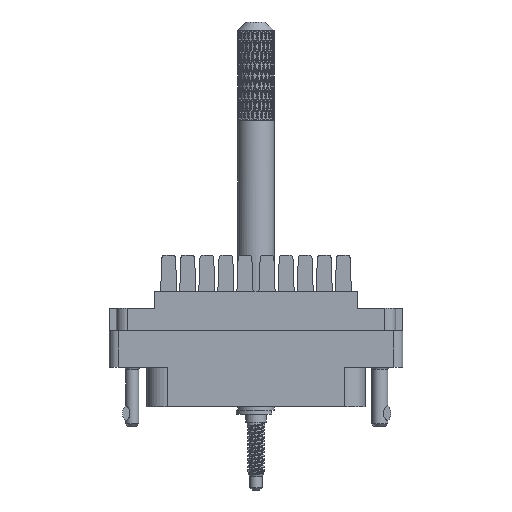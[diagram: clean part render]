
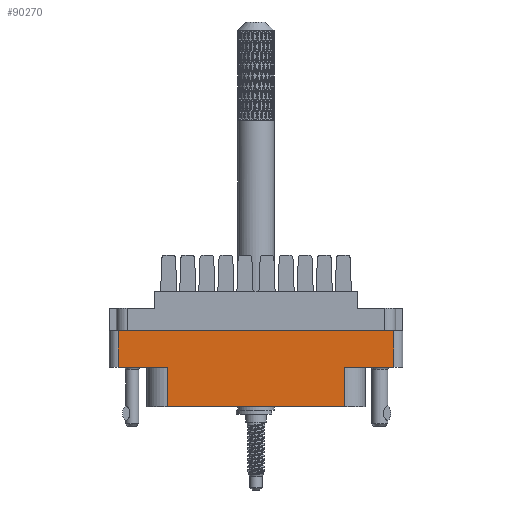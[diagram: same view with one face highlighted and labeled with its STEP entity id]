
A CAD part, front view. The second image highlights one B-rep face of the part: STEP entity #90270.
In plain terms, the highlighted planar face has unit normal (0, -1, 0).
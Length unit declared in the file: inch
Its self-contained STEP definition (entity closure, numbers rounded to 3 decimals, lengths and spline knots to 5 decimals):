
#3226 = EDGE_CURVE ( 'NONE', #63648, #46294, #106961, .T. ) ;
#3229 = VECTOR ( 'NONE', #85570, 39.37008 ) ;
#4358 = CARTESIAN_POINT ( 'NONE',  ( -1., -0.438, -0.789 ) ) ;
#5970 = DIRECTION ( 'NONE',  ( 0., -1., 0. ) ) ;
#6116 = LINE ( 'NONE', #42575, #76527 ) ;
#7362 = LINE ( 'NONE', #59778, #41862 ) ;
#9517 = CARTESIAN_POINT ( 'NONE',  ( 0.938, -0.438, -0.52 ) ) ;
#9749 = CARTESIAN_POINT ( 'NONE',  ( 0.938, -0.438, -0.268 ) ) ;
#12086 = VERTEX_POINT ( 'NONE', #44993 ) ;
#13782 = ORIENTED_EDGE ( 'NONE', *, *, #91361, .T. ) ;
#15289 = ORIENTED_EDGE ( 'NONE', *, *, #48787, .F. ) ;
#16369 = DIRECTION ( 'NONE',  ( 1., 0., 0. ) ) ;
#22045 = DIRECTION ( 'NONE',  ( 1., 0., 0. ) ) ;
#23377 = DIRECTION ( 'NONE',  ( 0., 0., 1. ) ) ;
#25219 = DIRECTION ( 'NONE',  ( 0., 0., -1. ) ) ;
#31307 = LINE ( 'NONE', #48378, #76660 ) ;
#32498 = CARTESIAN_POINT ( 'NONE',  ( -0.604, -0.438, -0.789 ) ) ;
#33995 = EDGE_CURVE ( 'NONE', #64044, #105680, #67907, .T. ) ;
#34691 = ORIENTED_EDGE ( 'NONE', *, *, #82466, .T. ) ;
#34885 = ORIENTED_EDGE ( 'NONE', *, *, #42756, .T. ) ;
#40197 = VECTOR ( 'NONE', #22045, 39.37008 ) ;
#41862 = VECTOR ( 'NONE', #23377, 39.37008 ) ;
#42575 = CARTESIAN_POINT ( 'NONE',  ( 0., -0.438, -0.52 ) ) ;
#42756 = EDGE_CURVE ( 'NONE', #12086, #107437, #6116, .T. ) ;
#44397 = EDGE_CURVE ( 'NONE', #80185, #12086, #31307, .T. ) ;
#44993 = CARTESIAN_POINT ( 'NONE',  ( -0.938, -0.438, -0.52 ) ) ;
#45252 = AXIS2_PLACEMENT_3D ( 'NONE', #84041, #5970, #102283 ) ;
#46294 = VERTEX_POINT ( 'NONE', #79488 ) ;
#48378 = CARTESIAN_POINT ( 'NONE',  ( -0.938, -0.438, -0.789 ) ) ;
#48787 = EDGE_CURVE ( 'NONE', #80185, #83169, #68099, .T. ) ;
#49274 = FACE_OUTER_BOUND ( 'NONE', #58283, .T. ) ;
#50682 = VECTOR ( 'NONE', #25219, 39.37008 ) ;
#53245 = CARTESIAN_POINT ( 'NONE',  ( -0.938, -0.438, -0.268 ) ) ;
#58283 = EDGE_LOOP ( 'NONE', ( #15289, #63528, #34885, #13782, #88174, #34691, #101642, #83854 ) ) ;
#58393 = DIRECTION ( 'NONE',  ( 1., 0., 0. ) ) ;
#58627 = CARTESIAN_POINT ( 'NONE',  ( 0.604, -0.438, -0.52 ) ) ;
#59778 = CARTESIAN_POINT ( 'NONE',  ( 0.938, -0.438, -0.789 ) ) ;
#61895 = EDGE_CURVE ( 'NONE', #64044, #83169, #7362, .T. ) ;
#63528 = ORIENTED_EDGE ( 'NONE', *, *, #44397, .T. ) ;
#63648 = VERTEX_POINT ( 'NONE', #32498 ) ;
#64044 = VERTEX_POINT ( 'NONE', #9517 ) ;
#66950 = PLANE ( 'NONE',  #45252 ) ;
#67907 = LINE ( 'NONE', #77565, #3229 ) ;
#68099 = LINE ( 'NONE', #112543, #89491 ) ;
#74106 = VECTOR ( 'NONE', #93405, 39.37008 ) ;
#76527 = VECTOR ( 'NONE', #16369, 39.37008 ) ;
#76660 = VECTOR ( 'NONE', #108253, 39.37008 ) ;
#77565 = CARTESIAN_POINT ( 'NONE',  ( 0., -0.438, -0.52 ) ) ;
#79488 = CARTESIAN_POINT ( 'NONE',  ( 0.604, -0.438, -0.789 ) ) ;
#80185 = VERTEX_POINT ( 'NONE', #53245 ) ;
#82466 = EDGE_CURVE ( 'NONE', #46294, #105680, #91723, .T. ) ;
#83169 = VERTEX_POINT ( 'NONE', #9749 ) ;
#83854 = ORIENTED_EDGE ( 'NONE', *, *, #61895, .T. ) ;
#84041 = CARTESIAN_POINT ( 'NONE',  ( -1., -0.438, -0.789 ) ) ;
#85570 = DIRECTION ( 'NONE',  ( -1., 0., 0. ) ) ;
#88174 = ORIENTED_EDGE ( 'NONE', *, *, #3226, .T. ) ;
#89491 = VECTOR ( 'NONE', #58393, 39.37008 ) ;
#90270 = ADVANCED_FACE ( 'NONE', ( #49274 ), #66950, .T. ) ;
#91361 = EDGE_CURVE ( 'NONE', #107437, #63648, #103294, .T. ) ;
#91723 = LINE ( 'NONE', #58627, #74106 ) ;
#93405 = DIRECTION ( 'NONE',  ( 0., 0., 1. ) ) ;
#94073 = CARTESIAN_POINT ( 'NONE',  ( -0.604, -0.438, -0.52 ) ) ;
#95362 = CARTESIAN_POINT ( 'NONE',  ( 0.604, -0.438, -0.52 ) ) ;
#101642 = ORIENTED_EDGE ( 'NONE', *, *, #33995, .F. ) ;
#102283 = DIRECTION ( 'NONE',  ( 0., 0., -1. ) ) ;
#103294 = LINE ( 'NONE', #108603, #50682 ) ;
#105680 = VERTEX_POINT ( 'NONE', #95362 ) ;
#106961 = LINE ( 'NONE', #4358, #40197 ) ;
#107437 = VERTEX_POINT ( 'NONE', #94073 ) ;
#108253 = DIRECTION ( 'NONE',  ( 0., 0., -1. ) ) ;
#108603 = CARTESIAN_POINT ( 'NONE',  ( -0.604, -0.438, -0.789 ) ) ;
#112543 = CARTESIAN_POINT ( 'NONE',  ( 0., -0.438, -0.268 ) ) ;
